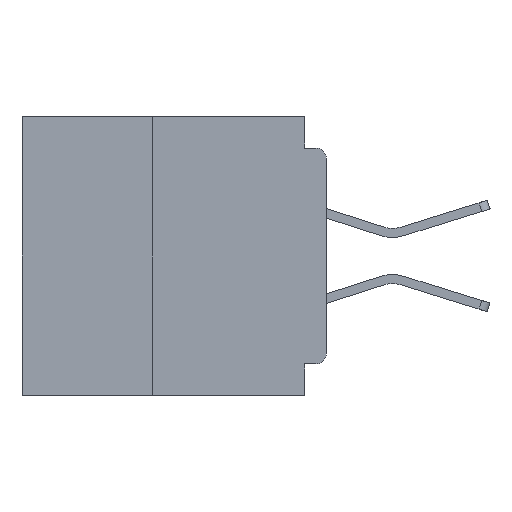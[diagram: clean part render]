
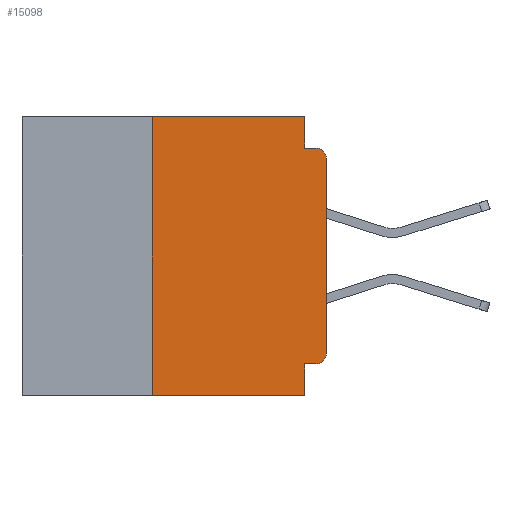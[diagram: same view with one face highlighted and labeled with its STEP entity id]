
A CAD part, left-side view. The second image highlights one B-rep face of the part: STEP entity #15098.
In plain terms, the highlighted planar face has unit normal (-1, 0, 0).
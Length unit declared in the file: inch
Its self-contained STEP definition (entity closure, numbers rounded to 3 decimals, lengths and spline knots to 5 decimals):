
#2632 = ORIENTED_EDGE ( 'NONE', *, *, #6305, .F. ) ;
#2929 = CIRCLE ( 'NONE', #26102, 0.015 ) ;
#3561 = DIRECTION ( 'NONE',  ( -1., 0., 0. ) ) ;
#4645 = ORIENTED_EDGE ( 'NONE', *, *, #36071, .T. ) ;
#4913 = ORIENTED_EDGE ( 'NONE', *, *, #18987, .T. ) ;
#5279 = VECTOR ( 'NONE', #36589, 39.37008 ) ;
#6305 = EDGE_CURVE ( 'NONE', #12461, #32382, #28743, .T. ) ;
#6555 = ORIENTED_EDGE ( 'NONE', *, *, #28582, .T. ) ;
#6571 = VERTEX_POINT ( 'NONE', #11188 ) ;
#6887 = CARTESIAN_POINT ( 'NONE',  ( 0., 0.437, 0. ) ) ;
#6892 = VECTOR ( 'NONE', #37679, 39.37008 ) ;
#7214 = EDGE_CURVE ( 'NONE', #32352, #22422, #34483, .T. ) ;
#7635 = AXIS2_PLACEMENT_3D ( 'NONE', #6887, #27822, #9901 ) ;
#7844 = CARTESIAN_POINT ( 'NONE',  ( 0., 0.031, 0. ) ) ;
#7908 = LINE ( 'NONE', #27820, #24861 ) ;
#9029 = FACE_OUTER_BOUND ( 'NONE', #22377, .T. ) ;
#9351 = ORIENTED_EDGE ( 'NONE', *, *, #33058, .F. ) ;
#9898 = DIRECTION ( 'NONE',  ( 0., -1., 0. ) ) ;
#9901 = DIRECTION ( 'NONE',  ( 0., 0., -1. ) ) ;
#10179 = CARTESIAN_POINT ( 'NONE',  ( 0., 0.015, -0.34 ) ) ;
#11037 = CARTESIAN_POINT ( 'NONE',  ( 0., 0., -0.045 ) ) ;
#11188 = CARTESIAN_POINT ( 'NONE',  ( 0., 0., -0.06 ) ) ;
#11389 = VECTOR ( 'NONE', #29518, 39.37008 ) ;
#11681 = CARTESIAN_POINT ( 'NONE',  ( 0., 0.015, -0.355 ) ) ;
#12461 = VERTEX_POINT ( 'NONE', #23778 ) ;
#13206 = DIRECTION ( 'NONE',  ( 0., 0., -1. ) ) ;
#13632 = VERTEX_POINT ( 'NONE', #26414 ) ;
#14218 = CARTESIAN_POINT ( 'NONE',  ( 0., 0.031, -0.045 ) ) ;
#14850 = LINE ( 'NONE', #20323, #6892 ) ;
#15098 = ADVANCED_FACE ( 'NONE', ( #9029 ), #36317, .F. ) ;
#15566 = CARTESIAN_POINT ( 'NONE',  ( 0., 0., -0.355 ) ) ;
#17251 = ORIENTED_EDGE ( 'NONE', *, *, #32170, .F. ) ;
#17924 = VERTEX_POINT ( 'NONE', #32181 ) ;
#18925 = VECTOR ( 'NONE', #19891, 39.37008 ) ;
#18987 = EDGE_CURVE ( 'NONE', #6571, #22422, #2929, .T. ) ;
#19503 = ORIENTED_EDGE ( 'NONE', *, *, #33766, .T. ) ;
#19554 = LINE ( 'NONE', #27372, #34158 ) ;
#19891 = DIRECTION ( 'NONE',  ( 0., -1., 0. ) ) ;
#20323 = CARTESIAN_POINT ( 'NONE',  ( 0., 0.031, -0.4 ) ) ;
#20913 = VECTOR ( 'NONE', #22634, 39.37008 ) ;
#21664 = CARTESIAN_POINT ( 'NONE',  ( 0., 0.015, -0.06 ) ) ;
#22377 = EDGE_LOOP ( 'NONE', ( #19503, #4913, #35968, #37329, #17251, #2632, #4645, #9351, #36987, #6555 ) ) ;
#22389 = CARTESIAN_POINT ( 'NONE',  ( 0., 0.25, -0.4 ) ) ;
#22422 = VERTEX_POINT ( 'NONE', #33985 ) ;
#22634 = DIRECTION ( 'NONE',  ( 0., 0., 1. ) ) ;
#23478 = CARTESIAN_POINT ( 'NONE',  ( 0., 0.25, 0. ) ) ;
#23608 = VECTOR ( 'NONE', #30453, 39.37008 ) ;
#23778 = CARTESIAN_POINT ( 'NONE',  ( 0., 0.25, -0.4 ) ) ;
#24536 = LINE ( 'NONE', #15566, #23608 ) ;
#24653 = DIRECTION ( 'NONE',  ( 0., 0., -1. ) ) ;
#24861 = VECTOR ( 'NONE', #9898, 39.37008 ) ;
#26102 = AXIS2_PLACEMENT_3D ( 'NONE', #21664, #3561, #24653 ) ;
#26414 = CARTESIAN_POINT ( 'NONE',  ( 0., 0.031, -0.355 ) ) ;
#27372 = CARTESIAN_POINT ( 'NONE',  ( 0., 0., 0. ) ) ;
#27558 = CARTESIAN_POINT ( 'NONE',  ( 0., 0.031, -0.4 ) ) ;
#27773 = VERTEX_POINT ( 'NONE', #11681 ) ;
#27820 = CARTESIAN_POINT ( 'NONE',  ( 0., 0.437, 0. ) ) ;
#27822 = DIRECTION ( 'NONE',  ( 1., 0., 0. ) ) ;
#27967 = CARTESIAN_POINT ( 'NONE',  ( 0., 0.437, -0.4 ) ) ;
#28582 = EDGE_CURVE ( 'NONE', #27773, #17924, #34133, .T. ) ;
#28743 = LINE ( 'NONE', #22389, #20913 ) ;
#29518 = DIRECTION ( 'NONE',  ( 0., 0., -1. ) ) ;
#30453 = DIRECTION ( 'NONE',  ( 0., 1., 0. ) ) ;
#30932 = DIRECTION ( 'NONE',  ( -1., 0., 0. ) ) ;
#31715 = VERTEX_POINT ( 'NONE', #7844 ) ;
#32123 = VERTEX_POINT ( 'NONE', #27558 ) ;
#32170 = EDGE_CURVE ( 'NONE', #32382, #31715, #7908, .T. ) ;
#32181 = CARTESIAN_POINT ( 'NONE',  ( 0., 0., -0.34 ) ) ;
#32352 = VERTEX_POINT ( 'NONE', #14218 ) ;
#32382 = VERTEX_POINT ( 'NONE', #23478 ) ;
#33058 = EDGE_CURVE ( 'NONE', #13632, #32123, #14850, .T. ) ;
#33766 = EDGE_CURVE ( 'NONE', #17924, #6571, #19554, .T. ) ;
#33985 = CARTESIAN_POINT ( 'NONE',  ( 0., 0.015, -0.045 ) ) ;
#34133 = CIRCLE ( 'NONE', #37209, 0.015 ) ;
#34158 = VECTOR ( 'NONE', #36005, 39.37008 ) ;
#34483 = LINE ( 'NONE', #11037, #18925 ) ;
#34913 = LINE ( 'NONE', #38010, #11389 ) ;
#35466 = EDGE_CURVE ( 'NONE', #31715, #32352, #34913, .T. ) ;
#35968 = ORIENTED_EDGE ( 'NONE', *, *, #7214, .F. ) ;
#35974 = EDGE_CURVE ( 'NONE', #27773, #13632, #24536, .T. ) ;
#36005 = DIRECTION ( 'NONE',  ( 0., 0., 1. ) ) ;
#36071 = EDGE_CURVE ( 'NONE', #12461, #32123, #36704, .T. ) ;
#36317 = PLANE ( 'NONE',  #7635 ) ;
#36589 = DIRECTION ( 'NONE',  ( 0., -1., 0. ) ) ;
#36704 = LINE ( 'NONE', #27967, #5279 ) ;
#36987 = ORIENTED_EDGE ( 'NONE', *, *, #35974, .F. ) ;
#37209 = AXIS2_PLACEMENT_3D ( 'NONE', #10179, #30932, #13206 ) ;
#37329 = ORIENTED_EDGE ( 'NONE', *, *, #35466, .F. ) ;
#37679 = DIRECTION ( 'NONE',  ( 0., 0., -1. ) ) ;
#38010 = CARTESIAN_POINT ( 'NONE',  ( 0., 0.031, 0. ) ) ;
